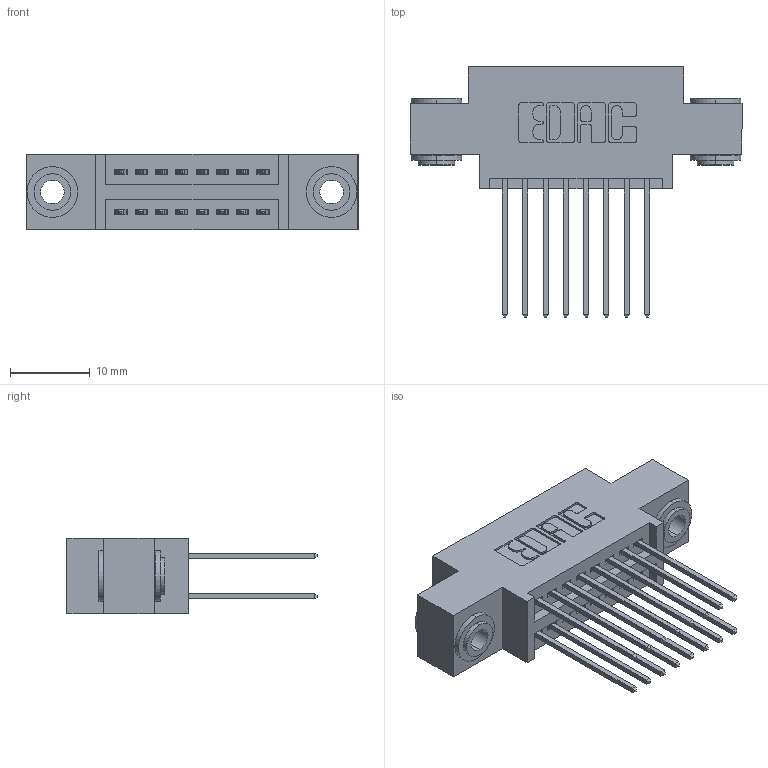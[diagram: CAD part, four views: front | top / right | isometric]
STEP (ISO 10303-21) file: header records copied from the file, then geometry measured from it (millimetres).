
FILE_DESCRIPTION (( 'STEP AP203' ), '1' );
FILE_NAME ('395-016-542-803.STEP', '2019-10-15T18:22:30', ( '' ), ( '' ), 'SwSTEP 2.0', 'SolidWorks 2016', '' );
FILE_SCHEMA (( 'CONFIG_CONTROL_DESIGN' ));
Length unit declared in the file: inch
Products named in the file (4): 395-016-542-803; 345 Part_0.170 Offset - 0.156 Dia-TH; 345-292-001_345-293-142; 345-250-002_345-250-002-102
Assembly tree (19 placements, depth 2):
  395-016-542-803
    345 Part_0.170 Offset - 0.156 Dia-TH
    345-292-001_345-293-142  x16
    345-250-002_345-250-002-102  x2
Bounding box: 41.53 x 31.29 x 9.4 mm (x, y, z)
Volume: 3699.2 mm3; surface area: 5506.4 mm2
Topology: 19 solids, 19 shells, 968 faces, 2813 edges, 1850 vertices
Faces by surface type: plane 622, cylinder 338, cone 8
Entity records: 11654 total; most frequent: CARTESIAN_POINT 1963, ORIENTED_EDGE 1890, DIRECTION 1803, EDGE_CURVE 945, VECTOR 757, LINE 757, VERTEX_POINT 626, AXIS2_PLACEMENT_3D 523
